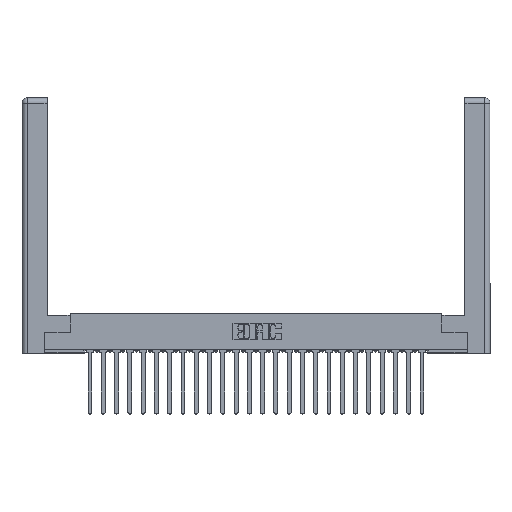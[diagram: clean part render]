
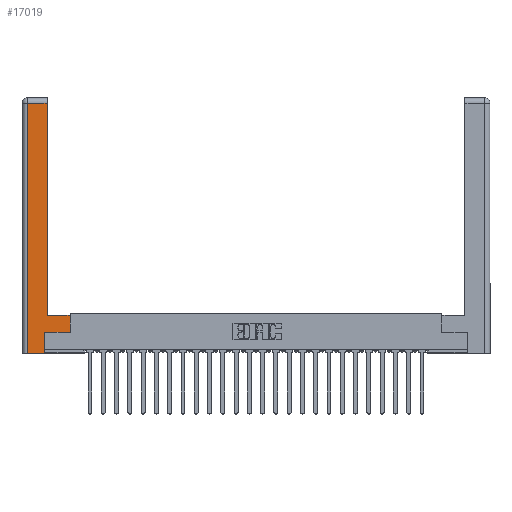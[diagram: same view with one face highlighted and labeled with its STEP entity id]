
A CAD part, top view. The second image highlights one B-rep face of the part: STEP entity #17019.
In plain terms, the highlighted planar face has unit normal (0, 0, 1).
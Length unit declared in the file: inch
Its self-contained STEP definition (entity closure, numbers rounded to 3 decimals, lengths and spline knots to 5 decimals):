
#408 = VECTOR ( 'NONE', #12728, 39.37008 ) ;
#1094 = EDGE_CURVE ( 'NONE', #20108, #3091, #7603, .T. ) ;
#2338 = VECTOR ( 'NONE', #6680, 39.37008 ) ;
#2417 = LINE ( 'NONE', #6099, #408 ) ;
#2604 = EDGE_CURVE ( 'NONE', #13590, #22865, #2417, .T. ) ;
#2652 = DIRECTION ( 'NONE',  ( -1., 0., 0. ) ) ;
#3091 = VERTEX_POINT ( 'NONE', #19157 ) ;
#3643 = VERTEX_POINT ( 'NONE', #12262 ) ;
#3685 = EDGE_CURVE ( 'NONE', #14983, #16086, #5702, .T. ) ;
#3803 = EDGE_CURVE ( 'NONE', #19431, #13590, #25791, .T. ) ;
#4340 = VECTOR ( 'NONE', #11231, 39.37008 ) ;
#4912 = AXIS2_PLACEMENT_3D ( 'NONE', #11341, #21858, #2652 ) ;
#5132 = EDGE_CURVE ( 'NONE', #3643, #14983, #18055, .T. ) ;
#5298 = CARTESIAN_POINT ( 'NONE',  ( 0.565, 0.245, 0. ) ) ;
#5702 = LINE ( 'NONE', #15300, #4340 ) ;
#6060 = ORIENTED_EDGE ( 'NONE', *, *, #3685, .T. ) ;
#6099 = CARTESIAN_POINT ( 'NONE',  ( 0.0615, 2.94, 0. ) ) ;
#6508 = CARTESIAN_POINT ( 'NONE',  ( 0.295, 0.45, 0. ) ) ;
#6680 = DIRECTION ( 'NONE',  ( 0., 1., 0. ) ) ;
#7161 = ORIENTED_EDGE ( 'NONE', *, *, #2604, .T. ) ;
#7444 = CARTESIAN_POINT ( 'NONE',  ( 0.265, 0.245, 0. ) ) ;
#7603 = LINE ( 'NONE', #26845, #19339 ) ;
#7998 = VECTOR ( 'NONE', #24202, 39.37008 ) ;
#8494 = ORIENTED_EDGE ( 'NONE', *, *, #1094, .T. ) ;
#8942 = LINE ( 'NONE', #7444, #11264 ) ;
#9349 = CARTESIAN_POINT ( 'NONE',  ( 0.0615, 2.94, 0. ) ) ;
#10397 = ORIENTED_EDGE ( 'NONE', *, *, #25464, .T. ) ;
#11231 = DIRECTION ( 'NONE',  ( 0., 1., 0. ) ) ;
#11264 = VECTOR ( 'NONE', #22247, 39.37008 ) ;
#11341 = CARTESIAN_POINT ( 'NONE',  ( 0., 0., 0. ) ) ;
#11867 = CARTESIAN_POINT ( 'NONE',  ( 0.295, 0.45, 0. ) ) ;
#12012 = CARTESIAN_POINT ( 'NONE',  ( 0.0615, 0., 0. ) ) ;
#12262 = CARTESIAN_POINT ( 'NONE',  ( 0.265, 0.245, 0. ) ) ;
#12728 = DIRECTION ( 'NONE',  ( -1., 0., 0. ) ) ;
#13323 = PLANE ( 'NONE',  #4912 ) ;
#13590 = VERTEX_POINT ( 'NONE', #21049 ) ;
#14033 = EDGE_CURVE ( 'NONE', #3091, #3643, #8942, .T. ) ;
#14948 = DIRECTION ( 'NONE',  ( -1., 0., 0. ) ) ;
#14983 = VERTEX_POINT ( 'NONE', #19401 ) ;
#15207 = CARTESIAN_POINT ( 'NONE',  ( 0.295, 3., 0. ) ) ;
#15300 = CARTESIAN_POINT ( 'NONE',  ( 0.565, 0.45, 0. ) ) ;
#15528 = DIRECTION ( 'NONE',  ( 0., -1., 0. ) ) ;
#16086 = VERTEX_POINT ( 'NONE', #20597 ) ;
#16199 = DIRECTION ( 'NONE',  ( 1., 0., 0. ) ) ;
#17019 = ADVANCED_FACE ( 'NONE', ( #17684 ), #13323, .F. ) ;
#17684 = FACE_OUTER_BOUND ( 'NONE', #18791, .T. ) ;
#18055 = LINE ( 'NONE', #5298, #7998 ) ;
#18332 = EDGE_CURVE ( 'NONE', #22865, #20108, #24643, .T. ) ;
#18791 = EDGE_LOOP ( 'NONE', ( #20820, #7161, #26178, #8494, #26937, #21373, #6060, #10397 ) ) ;
#19157 = CARTESIAN_POINT ( 'NONE',  ( 0.265, 0., 0. ) ) ;
#19339 = VECTOR ( 'NONE', #16199, 39.37008 ) ;
#19401 = CARTESIAN_POINT ( 'NONE',  ( 0.565, 0.245, 0. ) ) ;
#19431 = VERTEX_POINT ( 'NONE', #11867 ) ;
#20108 = VERTEX_POINT ( 'NONE', #12012 ) ;
#20597 = CARTESIAN_POINT ( 'NONE',  ( 0.565, 0.45, 0. ) ) ;
#20820 = ORIENTED_EDGE ( 'NONE', *, *, #3803, .T. ) ;
#21049 = CARTESIAN_POINT ( 'NONE',  ( 0.295, 2.94, 0. ) ) ;
#21373 = ORIENTED_EDGE ( 'NONE', *, *, #5132, .T. ) ;
#21858 = DIRECTION ( 'NONE',  ( 0., 0., -1. ) ) ;
#22247 = DIRECTION ( 'NONE',  ( 0., 1., 0. ) ) ;
#22546 = VECTOR ( 'NONE', #14948, 39.37008 ) ;
#22865 = VERTEX_POINT ( 'NONE', #9349 ) ;
#24202 = DIRECTION ( 'NONE',  ( 1., 0., 0. ) ) ;
#24643 = LINE ( 'NONE', #25991, #24971 ) ;
#24971 = VECTOR ( 'NONE', #15528, 39.37008 ) ;
#25464 = EDGE_CURVE ( 'NONE', #16086, #19431, #26201, .T. ) ;
#25791 = LINE ( 'NONE', #15207, #2338 ) ;
#25991 = CARTESIAN_POINT ( 'NONE',  ( 0.0615, 0., 0. ) ) ;
#26178 = ORIENTED_EDGE ( 'NONE', *, *, #18332, .T. ) ;
#26201 = LINE ( 'NONE', #6508, #22546 ) ;
#26845 = CARTESIAN_POINT ( 'NONE',  ( 0.265, 0., 0. ) ) ;
#26937 = ORIENTED_EDGE ( 'NONE', *, *, #14033, .T. ) ;
